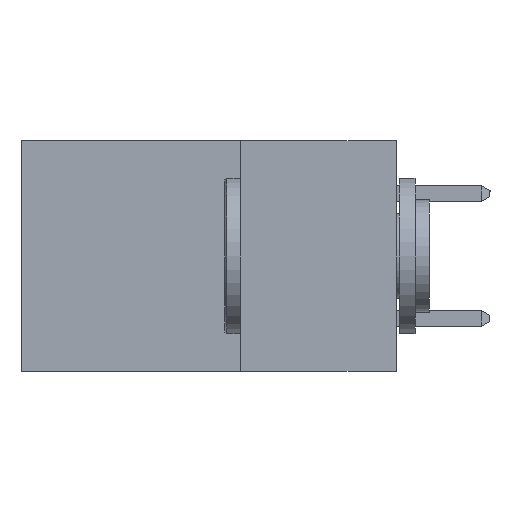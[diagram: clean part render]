
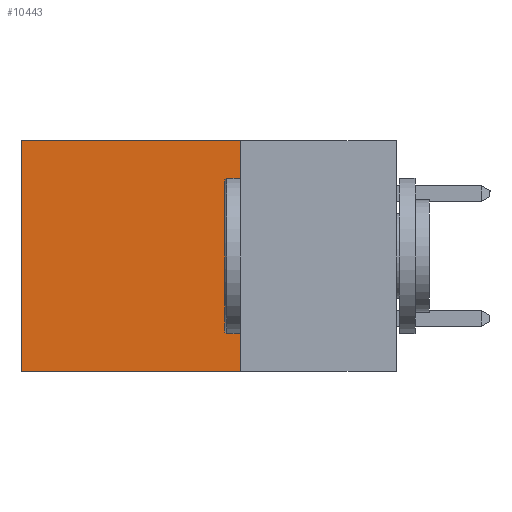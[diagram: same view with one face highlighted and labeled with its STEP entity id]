
A CAD part, left-side view. The second image highlights one B-rep face of the part: STEP entity #10443.
In plain terms, the highlighted planar face has unit normal (-1, 0, 0).
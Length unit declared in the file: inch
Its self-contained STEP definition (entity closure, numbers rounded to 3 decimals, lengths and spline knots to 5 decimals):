
#279 = VERTEX_POINT ( 'NONE', #19567 ) ;
#1151 = EDGE_CURVE ( 'NONE', #15671, #279, #6539, .T. ) ;
#2197 = CARTESIAN_POINT ( 'NONE',  ( 0.2615, 0.25, 0. ) ) ;
#3240 = DIRECTION ( 'NONE',  ( 0., 0., -1. ) ) ;
#3307 = PLANE ( 'NONE',  #13407 ) ;
#3714 = CARTESIAN_POINT ( 'NONE',  ( 0.2615, 0.6, 0. ) ) ;
#3765 = EDGE_LOOP ( 'NONE', ( #10737, #6016, #4315, #19804 ) ) ;
#4169 = LINE ( 'NONE', #18113, #8211 ) ;
#4315 = ORIENTED_EDGE ( 'NONE', *, *, #17113, .F. ) ;
#5036 = DIRECTION ( 'NONE',  ( 0., 1., 0. ) ) ;
#5925 = CARTESIAN_POINT ( 'NONE',  ( 0.2615, 0.25, -0.37 ) ) ;
#6016 = ORIENTED_EDGE ( 'NONE', *, *, #1151, .F. ) ;
#6539 = LINE ( 'NONE', #18913, #12117 ) ;
#7935 = CARTESIAN_POINT ( 'NONE',  ( 0.2615, 0.25, -0.37 ) ) ;
#7958 = LINE ( 'NONE', #14191, #15958 ) ;
#8211 = VECTOR ( 'NONE', #8594, 39.37008 ) ;
#8594 = DIRECTION ( 'NONE',  ( 0., 0., -1. ) ) ;
#10443 = ADVANCED_FACE ( 'NONE', ( #17172 ), #3307, .F. ) ;
#10737 = ORIENTED_EDGE ( 'NONE', *, *, #17436, .T. ) ;
#10749 = VECTOR ( 'NONE', #14569, 39.37008 ) ;
#12117 = VECTOR ( 'NONE', #5036, 39.37008 ) ;
#12306 = DIRECTION ( 'NONE',  ( 0., 0., -1. ) ) ;
#13258 = EDGE_CURVE ( 'NONE', #17903, #14624, #17867, .T. ) ;
#13407 = AXIS2_PLACEMENT_3D ( 'NONE', #7935, #14167, #12306 ) ;
#14167 = DIRECTION ( 'NONE',  ( 1., 0., 0. ) ) ;
#14191 = CARTESIAN_POINT ( 'NONE',  ( 0.2615, 0.6, -0.37 ) ) ;
#14569 = DIRECTION ( 'NONE',  ( 0., 1., 0. ) ) ;
#14624 = VERTEX_POINT ( 'NONE', #3714 ) ;
#15671 = VERTEX_POINT ( 'NONE', #5925 ) ;
#15958 = VECTOR ( 'NONE', #3240, 39.37008 ) ;
#17113 = EDGE_CURVE ( 'NONE', #17903, #15671, #4169, .T. ) ;
#17172 = FACE_OUTER_BOUND ( 'NONE', #3765, .T. ) ;
#17436 = EDGE_CURVE ( 'NONE', #14624, #279, #7958, .T. ) ;
#17652 = CARTESIAN_POINT ( 'NONE',  ( 0.2615, 0.25, 0. ) ) ;
#17867 = LINE ( 'NONE', #2197, #10749 ) ;
#17903 = VERTEX_POINT ( 'NONE', #17652 ) ;
#18113 = CARTESIAN_POINT ( 'NONE',  ( 0.2615, 0.25, -0.37 ) ) ;
#18913 = CARTESIAN_POINT ( 'NONE',  ( 0.2615, 0.25, -0.37 ) ) ;
#19567 = CARTESIAN_POINT ( 'NONE',  ( 0.2615, 0.6, -0.37 ) ) ;
#19804 = ORIENTED_EDGE ( 'NONE', *, *, #13258, .T. ) ;
